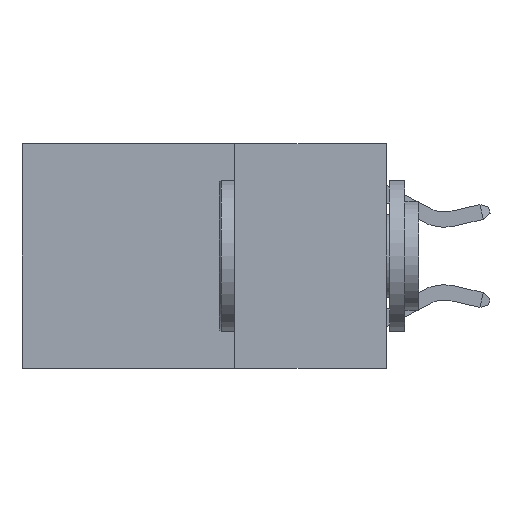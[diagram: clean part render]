
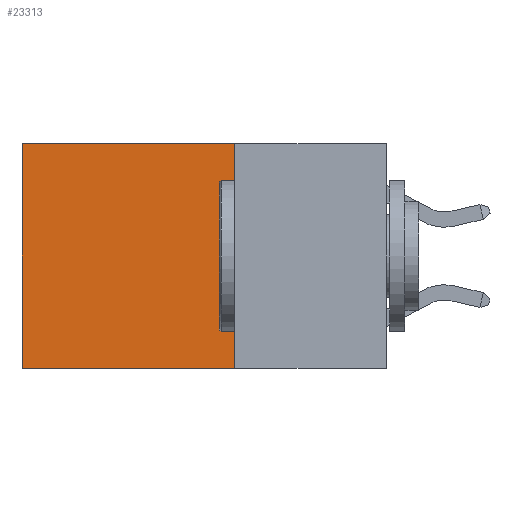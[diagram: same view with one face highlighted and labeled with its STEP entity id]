
A CAD part, left-side view. The second image highlights one B-rep face of the part: STEP entity #23313.
In plain terms, the highlighted planar face has unit normal (-1, 0, 0).
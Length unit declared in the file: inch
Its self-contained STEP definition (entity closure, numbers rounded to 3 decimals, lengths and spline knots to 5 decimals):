
#146 = VERTEX_POINT ( 'NONE', #24500 ) ;
#3073 = LINE ( 'NONE', #13008, #12693 ) ;
#3417 = DIRECTION ( 'NONE',  ( 0., 0., -1. ) ) ;
#3768 = EDGE_CURVE ( 'NONE', #18837, #146, #15021, .T. ) ;
#3821 = LINE ( 'NONE', #22558, #19054 ) ;
#4721 = CARTESIAN_POINT ( 'NONE',  ( 0.2625, 0.25, -0.37 ) ) ;
#6038 = DIRECTION ( 'NONE',  ( 1., 0., 0. ) ) ;
#6359 = EDGE_LOOP ( 'NONE', ( #16728, #10614, #18980, #15683 ) ) ;
#9387 = DIRECTION ( 'NONE',  ( 0., 1., 0. ) ) ;
#10045 = CARTESIAN_POINT ( 'NONE',  ( 0.2625, 0.6, 0. ) ) ;
#10360 = CARTESIAN_POINT ( 'NONE',  ( 0.2625, 0.6, -0.37 ) ) ;
#10614 = ORIENTED_EDGE ( 'NONE', *, *, #22432, .F. ) ;
#10779 = EDGE_CURVE ( 'NONE', #146, #22800, #22332, .T. ) ;
#11493 = DIRECTION ( 'NONE',  ( 0., 1., 0. ) ) ;
#11704 = VECTOR ( 'NONE', #11919, 39.37008 ) ;
#11919 = DIRECTION ( 'NONE',  ( 0., 0., -1. ) ) ;
#12115 = AXIS2_PLACEMENT_3D ( 'NONE', #17485, #6038, #19352 ) ;
#12693 = VECTOR ( 'NONE', #3417, 39.37008 ) ;
#13008 = CARTESIAN_POINT ( 'NONE',  ( 0.2625, 0.25, 0. ) ) ;
#13583 = VERTEX_POINT ( 'NONE', #4721 ) ;
#13777 = EDGE_CURVE ( 'NONE', #18837, #13583, #3073, .T. ) ;
#15021 = LINE ( 'NONE', #24651, #24380 ) ;
#15683 = ORIENTED_EDGE ( 'NONE', *, *, #3768, .T. ) ;
#16728 = ORIENTED_EDGE ( 'NONE', *, *, #10779, .T. ) ;
#17405 = PLANE ( 'NONE',  #12115 ) ;
#17485 = CARTESIAN_POINT ( 'NONE',  ( 0.2625, 0.25, 0. ) ) ;
#18837 = VERTEX_POINT ( 'NONE', #19664 ) ;
#18980 = ORIENTED_EDGE ( 'NONE', *, *, #13777, .F. ) ;
#19010 = FACE_OUTER_BOUND ( 'NONE', #6359, .T. ) ;
#19054 = VECTOR ( 'NONE', #9387, 39.37008 ) ;
#19352 = DIRECTION ( 'NONE',  ( 0., 0., -1. ) ) ;
#19664 = CARTESIAN_POINT ( 'NONE',  ( 0.2625, 0.25, 0. ) ) ;
#22332 = LINE ( 'NONE', #10045, #11704 ) ;
#22432 = EDGE_CURVE ( 'NONE', #13583, #22800, #3821, .T. ) ;
#22558 = CARTESIAN_POINT ( 'NONE',  ( 0.2625, 0.25, -0.37 ) ) ;
#22800 = VERTEX_POINT ( 'NONE', #10360 ) ;
#23313 = ADVANCED_FACE ( 'NONE', ( #19010 ), #17405, .F. ) ;
#24380 = VECTOR ( 'NONE', #11493, 39.37008 ) ;
#24500 = CARTESIAN_POINT ( 'NONE',  ( 0.2625, 0.6, 0. ) ) ;
#24651 = CARTESIAN_POINT ( 'NONE',  ( 0.2625, 0.25, 0. ) ) ;
